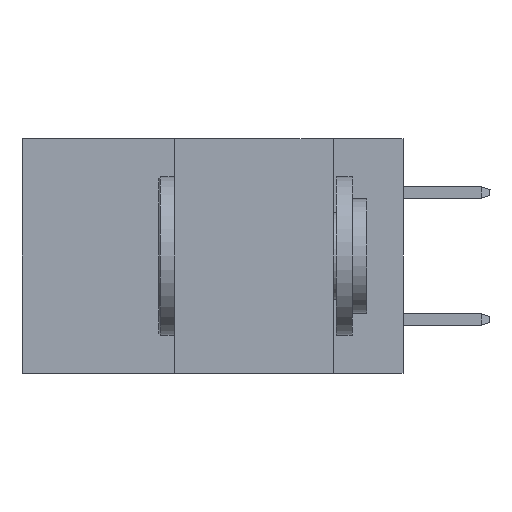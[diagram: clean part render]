
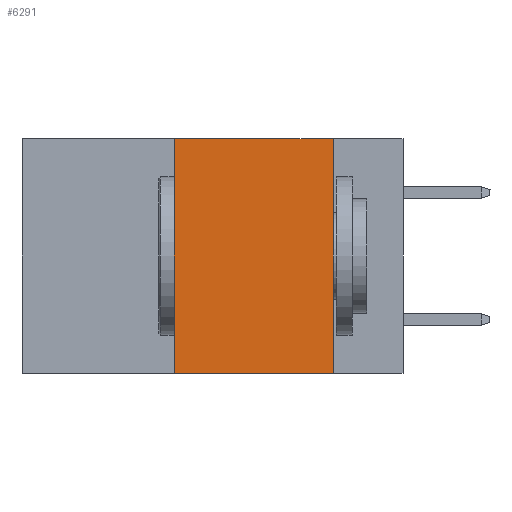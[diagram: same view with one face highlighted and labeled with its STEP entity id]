
A CAD part, left-side view. The second image highlights one B-rep face of the part: STEP entity #6291.
In plain terms, the highlighted planar face has unit normal (-1, 0, 0).
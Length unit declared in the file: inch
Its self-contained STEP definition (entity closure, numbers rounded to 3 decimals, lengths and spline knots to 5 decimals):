
#3483 = CARTESIAN_POINT ( 'NONE',  ( 0., 0.36, -0.37 ) ) ;
#3933 = EDGE_LOOP ( 'NONE', ( #13812, #9744, #4699, #20284 ) ) ;
#4167 = VERTEX_POINT ( 'NONE', #26346 ) ;
#4335 = CARTESIAN_POINT ( 'NONE',  ( 0., 0.36, 0. ) ) ;
#4699 = ORIENTED_EDGE ( 'NONE', *, *, #35771, .F. ) ;
#4809 = CARTESIAN_POINT ( 'NONE',  ( 0., 0.6, -0.37 ) ) ;
#4976 = LINE ( 'NONE', #4809, #33717 ) ;
#6104 = VECTOR ( 'NONE', #10291, 39.37008 ) ;
#6291 = ADVANCED_FACE ( 'NONE', ( #17112 ), #16938, .F. ) ;
#8705 = LINE ( 'NONE', #20361, #19658 ) ;
#9744 = ORIENTED_EDGE ( 'NONE', *, *, #19780, .F. ) ;
#10291 = DIRECTION ( 'NONE',  ( 0., -1., 0. ) ) ;
#13371 = VERTEX_POINT ( 'NONE', #4335 ) ;
#13812 = ORIENTED_EDGE ( 'NONE', *, *, #32454, .F. ) ;
#14481 = CARTESIAN_POINT ( 'NONE',  ( 0., 0.11, 0. ) ) ;
#16612 = DIRECTION ( 'NONE',  ( 0., -1., 0. ) ) ;
#16938 = PLANE ( 'NONE',  #37038 ) ;
#17112 = FACE_OUTER_BOUND ( 'NONE', #3933, .T. ) ;
#19658 = VECTOR ( 'NONE', #37384, 39.37008 ) ;
#19780 = EDGE_CURVE ( 'NONE', #13371, #24281, #37212, .T. ) ;
#20284 = ORIENTED_EDGE ( 'NONE', *, *, #21500, .T. ) ;
#20361 = CARTESIAN_POINT ( 'NONE',  ( 0., 0.36, 0. ) ) ;
#21500 = EDGE_CURVE ( 'NONE', #30358, #4167, #4976, .T. ) ;
#22110 = CARTESIAN_POINT ( 'NONE',  ( 0., 0.6, 0. ) ) ;
#22427 = VECTOR ( 'NONE', #35127, 39.37008 ) ;
#24281 = VERTEX_POINT ( 'NONE', #26917 ) ;
#26102 = CARTESIAN_POINT ( 'NONE',  ( 0., 0.6, 0. ) ) ;
#26346 = CARTESIAN_POINT ( 'NONE',  ( 0., 0.11, -0.37 ) ) ;
#26917 = CARTESIAN_POINT ( 'NONE',  ( 0., 0.11, 0. ) ) ;
#28775 = DIRECTION ( 'NONE',  ( 0., 0., -1. ) ) ;
#29765 = LINE ( 'NONE', #14481, #22427 ) ;
#30358 = VERTEX_POINT ( 'NONE', #3483 ) ;
#31658 = DIRECTION ( 'NONE',  ( 1., 0., 0. ) ) ;
#32454 = EDGE_CURVE ( 'NONE', #24281, #4167, #29765, .T. ) ;
#33717 = VECTOR ( 'NONE', #16612, 39.37008 ) ;
#35127 = DIRECTION ( 'NONE',  ( 0., 0., -1. ) ) ;
#35771 = EDGE_CURVE ( 'NONE', #30358, #13371, #8705, .T. ) ;
#37038 = AXIS2_PLACEMENT_3D ( 'NONE', #26102, #31658, #28775 ) ;
#37212 = LINE ( 'NONE', #22110, #6104 ) ;
#37384 = DIRECTION ( 'NONE',  ( 0., 0., 1. ) ) ;
